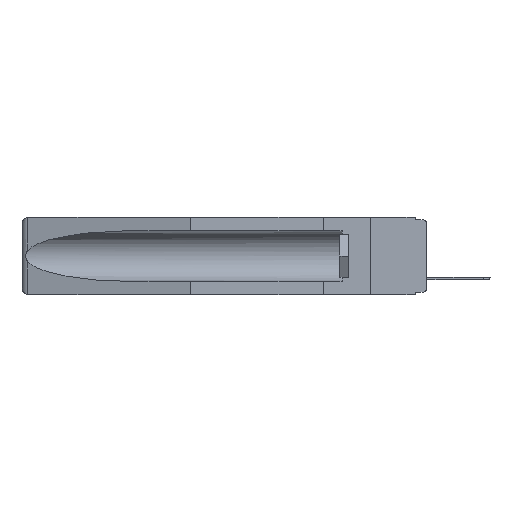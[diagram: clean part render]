
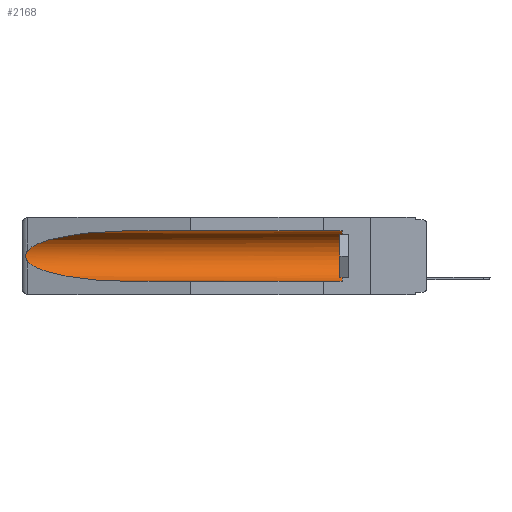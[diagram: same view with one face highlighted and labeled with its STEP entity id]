
A CAD part, left-side view. The second image highlights one B-rep face of the part: STEP entity #2168.
In plain terms, the highlighted cylindrical face has radius 2.857 mm (diameter 5.715 mm), a partial arc.
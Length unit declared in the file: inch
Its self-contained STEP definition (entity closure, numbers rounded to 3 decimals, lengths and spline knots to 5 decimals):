
#36 = ORIENTED_EDGE ( 'NONE', *, *, #6830, .T. ) ;
#340 = DIRECTION ( 'NONE',  ( 0., 0., 1. ) ) ;
#768 = DIRECTION ( 'NONE',  ( 0., 0., 1. ) ) ;
#1204 = CARTESIAN_POINT ( 'NONE',  ( 0.26537, 1.52718, -0.14972 ) ) ;
#1672 = ORIENTED_EDGE ( 'NONE', *, *, #1783, .F. ) ;
#1783 = EDGE_CURVE ( 'NONE', #15755, #11623, #3569, .T. ) ;
#2020 = ORIENTED_EDGE ( 'NONE', *, *, #6501, .T. ) ;
#2094 = ORIENTED_EDGE ( 'NONE', *, *, #5653, .T. ) ;
#2155 = CARTESIAN_POINT ( 'NONE',  ( 0.155, -0.30754, -0.1715 ) ) ;
#2168 = ADVANCED_FACE ( 'NONE', ( #13976 ), #16396, .F. ) ;
#3145 = CARTESIAN_POINT ( 'NONE',  ( 0.155, 1.07973, -0.059 ) ) ;
#3569 = LINE ( 'NONE', #11482, #8921 ) ;
#3641 = EDGE_CURVE ( 'NONE', #12060, #5483, #10621, .T. ) ;
#4112 = ORIENTED_EDGE ( 'NONE', *, *, #3641, .T. ) ;
#4244 = CARTESIAN_POINT ( 'NONE',  ( 0.21114, 1.30732, -0.284 ) ) ;
#4363 = AXIS2_PLACEMENT_3D ( 'NONE', #2155, #12752, #768 ) ;
#4923 = CARTESIAN_POINT ( 'NONE',  ( 0.2673, 1.5327, -0.16383 ) ) ;
#5024 = CARTESIAN_POINT ( 'NONE',  ( 0.21114, 1.30732, -0.059 ) ) ;
#5100 = CARTESIAN_POINT ( 'NONE',  ( 0.2673, 1.53269, -0.17917 ) ) ;
#5229 = DIRECTION ( 'NONE',  ( 0., 1., 0. ) ) ;
#5483 = VERTEX_POINT ( 'NONE', #16216 ) ;
#5653 = EDGE_CURVE ( 'NONE', #7178, #13663, #6146, .T. ) ;
#5874 = CARTESIAN_POINT ( 'NONE',  ( 0.155, 0.126, -0.284 ) ) ;
#5921 = DIRECTION ( 'NONE',  ( 0., 1., 0. ) ) ;
#6146 = LINE ( 'NONE', #16177, #10830 ) ;
#6420 = CARTESIAN_POINT ( 'NONE',  ( 0.25451, 1.48313, -0.09465 ) ) ;
#6501 = EDGE_CURVE ( 'NONE', #13663, #12060, #7293, .T. ) ;
#6830 = EDGE_CURVE ( 'NONE', #15755, #7178, #14735, .T. ) ;
#7178 = VERTEX_POINT ( 'NONE', #13431 ) ;
#7293 =( BOUNDED_CURVE ( )  B_SPLINE_CURVE ( 3, ( #16915, #5024, #6420, #15538 ),
 .UNSPECIFIED., .F., .T. ) 
 B_SPLINE_CURVE_WITH_KNOTS ( ( 4, 4 ),
 ( 4.71239, 6.08839 ),
 .UNSPECIFIED. ) 
 CURVE ( )  GEOMETRIC_REPRESENTATION_ITEM ( )  RATIONAL_B_SPLINE_CURVE ( ( 1., 0.848, 0.848, 1. ) ) 
 REPRESENTATION_ITEM ( '' )  );
#7374 = CARTESIAN_POINT ( 'NONE',  ( 0.26537, 1.52718, -0.14972 ) ) ;
#7643 = CARTESIAN_POINT ( 'NONE',  ( 0.26597, 1.52961, -0.15275 ) ) ;
#7809 = CARTESIAN_POINT ( 'NONE',  ( 0.26655, 1.53094, -0.18657 ) ) ;
#7970 = CARTESIAN_POINT ( 'NONE',  ( 0.2675, 1.53308, -0.17534 ) ) ;
#8243 = CARTESIAN_POINT ( 'NONE',  ( 0.155, 0.126, -0.1715 ) ) ;
#8921 = VECTOR ( 'NONE', #5921, 39.37008 ) ;
#9546 = CARTESIAN_POINT ( 'NONE',  ( 0.155, 1.07973, -0.284 ) ) ;
#9632 = EDGE_LOOP ( 'NONE', ( #2020, #4112, #13965, #1672, #36, #2094 ) ) ;
#9749 = AXIS2_PLACEMENT_3D ( 'NONE', #8243, #13622, #340 ) ;
#10231 = CARTESIAN_POINT ( 'NONE',  ( 0.26597, 1.5296, -0.19026 ) ) ;
#10621 = B_SPLINE_CURVE_WITH_KNOTS ( 'NONE', 3,
 ( #1204, #7643, #16903, #4923, #13185, #7970, #5100, #7809, #10231, #11618 ),
 .UNSPECIFIED., .F., .F.,
 ( 4, 2, 2, 2, 4 ),
 ( 0., 0.00029, 0.00058, 0.00087, 0.00117 ),
 .UNSPECIFIED. ) ;
#10830 = VECTOR ( 'NONE', #5229, 39.37008 ) ;
#11482 = CARTESIAN_POINT ( 'NONE',  ( 0.155, -0.30754, -0.284 ) ) ;
#11618 = CARTESIAN_POINT ( 'NONE',  ( 0.26537, 1.52718, -0.19328 ) ) ;
#11623 = VERTEX_POINT ( 'NONE', #16913 ) ;
#11844 =( BOUNDED_CURVE ( )  B_SPLINE_CURVE ( 3, ( #11984, #16133, #4244, #9546 ),
 .UNSPECIFIED., .F., .T. ) 
 B_SPLINE_CURVE_WITH_KNOTS ( ( 4, 4 ),
 ( 0.1948, 1.5708 ),
 .UNSPECIFIED. ) 
 CURVE ( )  GEOMETRIC_REPRESENTATION_ITEM ( )  RATIONAL_B_SPLINE_CURVE ( ( 1., 0.848, 0.848, 1. ) ) 
 REPRESENTATION_ITEM ( '' )  );
#11984 = CARTESIAN_POINT ( 'NONE',  ( 0.26537, 1.52718, -0.19328 ) ) ;
#12060 = VERTEX_POINT ( 'NONE', #7374 ) ;
#12752 = DIRECTION ( 'NONE',  ( 0., 1., 0. ) ) ;
#13185 = CARTESIAN_POINT ( 'NONE',  ( 0.2675, 1.53308, -0.16763 ) ) ;
#13431 = CARTESIAN_POINT ( 'NONE',  ( 0.155, 0.126, -0.059 ) ) ;
#13622 = DIRECTION ( 'NONE',  ( 0., -1., 0. ) ) ;
#13663 = VERTEX_POINT ( 'NONE', #3145 ) ;
#13965 = ORIENTED_EDGE ( 'NONE', *, *, #14035, .T. ) ;
#13976 = FACE_OUTER_BOUND ( 'NONE', #9632, .T. ) ;
#14035 = EDGE_CURVE ( 'NONE', #5483, #11623, #11844, .T. ) ;
#14735 = CIRCLE ( 'NONE', #9749, 0.1125 ) ;
#15538 = CARTESIAN_POINT ( 'NONE',  ( 0.26537, 1.52718, -0.14972 ) ) ;
#15755 = VERTEX_POINT ( 'NONE', #5874 ) ;
#16133 = CARTESIAN_POINT ( 'NONE',  ( 0.25451, 1.48313, -0.24835 ) ) ;
#16177 = CARTESIAN_POINT ( 'NONE',  ( 0.155, -0.30754, -0.059 ) ) ;
#16216 = CARTESIAN_POINT ( 'NONE',  ( 0.26537, 1.52718, -0.19328 ) ) ;
#16396 = CYLINDRICAL_SURFACE ( 'NONE', #4363, 0.1125 ) ;
#16903 = CARTESIAN_POINT ( 'NONE',  ( 0.26654, 1.53092, -0.15636 ) ) ;
#16913 = CARTESIAN_POINT ( 'NONE',  ( 0.155, 1.07973, -0.284 ) ) ;
#16915 = CARTESIAN_POINT ( 'NONE',  ( 0.155, 1.07973, -0.059 ) ) ;
